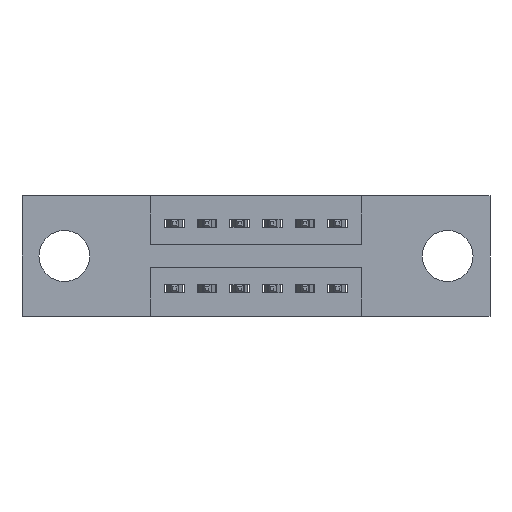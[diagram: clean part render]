
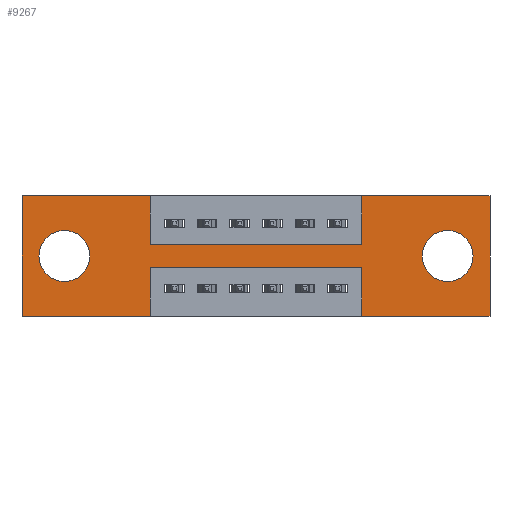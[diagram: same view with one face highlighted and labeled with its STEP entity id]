
A CAD part, front view. The second image highlights one B-rep face of the part: STEP entity #9267.
In plain terms, the highlighted planar face has unit normal (0, -1, 0).
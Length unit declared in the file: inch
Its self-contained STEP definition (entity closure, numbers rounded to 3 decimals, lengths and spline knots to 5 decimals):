
#48 = EDGE_CURVE ( 'NONE', #7557, #5748, #2811, .T. ) ;
#67 = VERTEX_POINT ( 'NONE', #7478 ) ;
#99 = CARTESIAN_POINT ( 'NONE',  ( 0.3925, 0., 0. ) ) ;
#115 = ORIENTED_EDGE ( 'NONE', *, *, #48, .F. ) ;
#135 = VERTEX_POINT ( 'NONE', #356 ) ;
#152 = EDGE_CURVE ( 'NONE', #9398, #7229, #5936, .T. ) ;
#356 = CARTESIAN_POINT ( 'NONE',  ( 0., 0., -0.37 ) ) ;
#578 = VERTEX_POINT ( 'NONE', #6180 ) ;
#628 = ORIENTED_EDGE ( 'NONE', *, *, #1467, .F. ) ;
#659 = DIRECTION ( 'NONE',  ( 0., 0., -1. ) ) ;
#693 = VECTOR ( 'NONE', #9551, 39.37008 ) ;
#712 = ORIENTED_EDGE ( 'NONE', *, *, #730, .T. ) ;
#730 = EDGE_CURVE ( 'NONE', #5898, #7509, #4365, .T. ) ;
#741 = VERTEX_POINT ( 'NONE', #99 ) ;
#786 = EDGE_CURVE ( 'NONE', #741, #578, #2182, .T. ) ;
#837 = DIRECTION ( 'NONE',  ( 0., 0., -1. ) ) ;
#884 = VERTEX_POINT ( 'NONE', #7460 ) ;
#1011 = LINE ( 'NONE', #1949, #693 ) ;
#1019 = LINE ( 'NONE', #2818, #8676 ) ;
#1350 = LINE ( 'NONE', #1994, #3423 ) ;
#1365 = VERTEX_POINT ( 'NONE', #2660 ) ;
#1382 = DIRECTION ( 'NONE',  ( 0., 0., 1. ) ) ;
#1467 = EDGE_CURVE ( 'NONE', #1818, #7557, #5525, .T. ) ;
#1524 = ORIENTED_EDGE ( 'NONE', *, *, #2835, .F. ) ;
#1645 = EDGE_CURVE ( 'NONE', #9322, #135, #4578, .T. ) ;
#1724 = CIRCLE ( 'NONE', #9318, 0.078 ) ;
#1818 = VERTEX_POINT ( 'NONE', #3480 ) ;
#1949 = CARTESIAN_POINT ( 'NONE',  ( 0.3925, 0., -0.22 ) ) ;
#1976 = DIRECTION ( 'NONE',  ( 1., 0., 0. ) ) ;
#1994 = CARTESIAN_POINT ( 'NONE',  ( 0.3925, 0., -0.37 ) ) ;
#2040 = DIRECTION ( 'NONE',  ( 1., 0., 0. ) ) ;
#2086 = DIRECTION ( 'NONE',  ( 0., 0., -1. ) ) ;
#2177 = EDGE_CURVE ( 'NONE', #135, #5758, #5167, .T. ) ;
#2182 = LINE ( 'NONE', #6666, #4133 ) ;
#2308 = CARTESIAN_POINT ( 'NONE',  ( 0., 0., 0. ) ) ;
#2323 = EDGE_CURVE ( 'NONE', #67, #9322, #1350, .T. ) ;
#2373 = AXIS2_PLACEMENT_3D ( 'NONE', #4329, #8053, #5105 ) ;
#2604 = LINE ( 'NONE', #6852, #7099 ) ;
#2633 = CARTESIAN_POINT ( 'NONE',  ( 1.435, 0., 0. ) ) ;
#2660 = CARTESIAN_POINT ( 'NONE',  ( 1.0425, 0., -0.22 ) ) ;
#2692 = CARTESIAN_POINT ( 'NONE',  ( 1.0425, 0., 0. ) ) ;
#2811 = LINE ( 'NONE', #8893, #7665 ) ;
#2818 = CARTESIAN_POINT ( 'NONE',  ( 0., 0., 0. ) ) ;
#2835 = EDGE_CURVE ( 'NONE', #6973, #884, #2604, .T. ) ;
#2857 = ORIENTED_EDGE ( 'NONE', *, *, #4338, .F. ) ;
#2935 = ORIENTED_EDGE ( 'NONE', *, *, #786, .F. ) ;
#2946 = DIRECTION ( 'NONE',  ( 0., 0., 1. ) ) ;
#3013 = EDGE_CURVE ( 'NONE', #7509, #5898, #3643, .T. ) ;
#3135 = LINE ( 'NONE', #7238, #6815 ) ;
#3232 = ORIENTED_EDGE ( 'NONE', *, *, #7795, .F. ) ;
#3386 = CARTESIAN_POINT ( 'NONE',  ( 1.305, 0., -0.107 ) ) ;
#3423 = VECTOR ( 'NONE', #2086, 39.37008 ) ;
#3480 = CARTESIAN_POINT ( 'NONE',  ( 1.0425, 0., -0.15 ) ) ;
#3643 = CIRCLE ( 'NONE', #6067, 0.078 ) ;
#3680 = DIRECTION ( 'NONE',  ( 0., 1., 0. ) ) ;
#3715 = DIRECTION ( 'NONE',  ( 0., 0., -1. ) ) ;
#3824 = DIRECTION ( 'NONE',  ( -1., 0., 0. ) ) ;
#4133 = VECTOR ( 'NONE', #3715, 39.37008 ) ;
#4143 = ORIENTED_EDGE ( 'NONE', *, *, #2323, .F. ) ;
#4182 = AXIS2_PLACEMENT_3D ( 'NONE', #8421, #3680, #2946 ) ;
#4199 = CARTESIAN_POINT ( 'NONE',  ( 1.435, 0., -0.37 ) ) ;
#4212 = FACE_OUTER_BOUND ( 'NONE', #9157, .T. ) ;
#4271 = ORIENTED_EDGE ( 'NONE', *, *, #2177, .F. ) ;
#4310 = CARTESIAN_POINT ( 'NONE',  ( 0.3925, 0., -0.15 ) ) ;
#4329 = CARTESIAN_POINT ( 'NONE',  ( 0., 0., -0.37 ) ) ;
#4333 = FACE_BOUND ( 'NONE', #7493, .T. ) ;
#4338 = EDGE_CURVE ( 'NONE', #884, #1365, #7189, .T. ) ;
#4365 = CIRCLE ( 'NONE', #4182, 0.078 ) ;
#4370 = VECTOR ( 'NONE', #2040, 39.37008 ) ;
#4402 = ORIENTED_EDGE ( 'NONE', *, *, #6558, .F. ) ;
#4446 = DIRECTION ( 'NONE',  ( 1., 0., 0. ) ) ;
#4565 = DIRECTION ( 'NONE',  ( 0., 0., 1. ) ) ;
#4578 = LINE ( 'NONE', #6000, #6687 ) ;
#5061 = FACE_BOUND ( 'NONE', #6332, .T. ) ;
#5105 = DIRECTION ( 'NONE',  ( 0., 0., -1. ) ) ;
#5167 = LINE ( 'NONE', #2308, #6774 ) ;
#5267 = DIRECTION ( 'NONE',  ( 0., 1., 0. ) ) ;
#5436 = CARTESIAN_POINT ( 'NONE',  ( 0.3925, 0., -0.37 ) ) ;
#5525 = LINE ( 'NONE', #6208, #7719 ) ;
#5537 = CARTESIAN_POINT ( 'NONE',  ( 0.13, 0., -0.185 ) ) ;
#5595 = DIRECTION ( 'NONE',  ( 0., 0., 1. ) ) ;
#5748 = VERTEX_POINT ( 'NONE', #2633 ) ;
#5758 = VERTEX_POINT ( 'NONE', #9236 ) ;
#5898 = VERTEX_POINT ( 'NONE', #6348 ) ;
#5936 = CIRCLE ( 'NONE', #8399, 0.078 ) ;
#6000 = CARTESIAN_POINT ( 'NONE',  ( 0., 0., -0.37 ) ) ;
#6039 = EDGE_CURVE ( 'NONE', #5748, #6973, #3135, .T. ) ;
#6067 = AXIS2_PLACEMENT_3D ( 'NONE', #5537, #8468, #5595 ) ;
#6165 = ORIENTED_EDGE ( 'NONE', *, *, #6039, .F. ) ;
#6180 = CARTESIAN_POINT ( 'NONE',  ( 0.3925, 0., -0.15 ) ) ;
#6208 = CARTESIAN_POINT ( 'NONE',  ( 1.0425, 0., 0. ) ) ;
#6332 = EDGE_LOOP ( 'NONE', ( #712, #9542 ) ) ;
#6348 = CARTESIAN_POINT ( 'NONE',  ( 0.13, 0., -0.107 ) ) ;
#6393 = VECTOR ( 'NONE', #1382, 39.37008 ) ;
#6468 = LINE ( 'NONE', #4310, #4370 ) ;
#6513 = ORIENTED_EDGE ( 'NONE', *, *, #1645, .F. ) ;
#6543 = EDGE_CURVE ( 'NONE', #578, #1818, #6468, .T. ) ;
#6558 = EDGE_CURVE ( 'NONE', #5758, #741, #1019, .T. ) ;
#6666 = CARTESIAN_POINT ( 'NONE',  ( 0.3925, 0., 0. ) ) ;
#6687 = VECTOR ( 'NONE', #3824, 39.37008 ) ;
#6712 = EDGE_CURVE ( 'NONE', #7229, #9398, #1724, .T. ) ;
#6774 = VECTOR ( 'NONE', #4565, 39.37008 ) ;
#6815 = VECTOR ( 'NONE', #7306, 39.37008 ) ;
#6852 = CARTESIAN_POINT ( 'NONE',  ( 0., 0., -0.37 ) ) ;
#6874 = DIRECTION ( 'NONE',  ( 0., 0., 1. ) ) ;
#6973 = VERTEX_POINT ( 'NONE', #4199 ) ;
#7099 = VECTOR ( 'NONE', #8408, 39.37008 ) ;
#7189 = LINE ( 'NONE', #8746, #6393 ) ;
#7229 = VERTEX_POINT ( 'NONE', #8800 ) ;
#7238 = CARTESIAN_POINT ( 'NONE',  ( 1.435, 0., 0. ) ) ;
#7306 = DIRECTION ( 'NONE',  ( 0., 0., -1. ) ) ;
#7351 = DIRECTION ( 'NONE',  ( 0., 1., 0. ) ) ;
#7460 = CARTESIAN_POINT ( 'NONE',  ( 1.0425, 0., -0.37 ) ) ;
#7478 = CARTESIAN_POINT ( 'NONE',  ( 0.3925, 0., -0.22 ) ) ;
#7493 = EDGE_LOOP ( 'NONE', ( #9545, #8332 ) ) ;
#7509 = VERTEX_POINT ( 'NONE', #9256 ) ;
#7520 = ORIENTED_EDGE ( 'NONE', *, *, #6543, .F. ) ;
#7557 = VERTEX_POINT ( 'NONE', #2692 ) ;
#7665 = VECTOR ( 'NONE', #4446, 39.37008 ) ;
#7719 = VECTOR ( 'NONE', #6874, 39.37008 ) ;
#7795 = EDGE_CURVE ( 'NONE', #1365, #67, #1011, .T. ) ;
#8053 = DIRECTION ( 'NONE',  ( 0., -1., 0. ) ) ;
#8332 = ORIENTED_EDGE ( 'NONE', *, *, #6712, .T. ) ;
#8399 = AXIS2_PLACEMENT_3D ( 'NONE', #8961, #5267, #837 ) ;
#8408 = DIRECTION ( 'NONE',  ( -1., 0., 0. ) ) ;
#8421 = CARTESIAN_POINT ( 'NONE',  ( 0.13, 0., -0.185 ) ) ;
#8468 = DIRECTION ( 'NONE',  ( 0., 1., 0. ) ) ;
#8676 = VECTOR ( 'NONE', #1976, 39.37008 ) ;
#8746 = CARTESIAN_POINT ( 'NONE',  ( 1.0425, 0., -0.37 ) ) ;
#8799 = CARTESIAN_POINT ( 'NONE',  ( 1.305, 0., -0.185 ) ) ;
#8800 = CARTESIAN_POINT ( 'NONE',  ( 1.305, 0., -0.263 ) ) ;
#8893 = CARTESIAN_POINT ( 'NONE',  ( 0., 0., 0. ) ) ;
#8961 = CARTESIAN_POINT ( 'NONE',  ( 1.305, 0., -0.185 ) ) ;
#9157 = EDGE_LOOP ( 'NONE', ( #4143, #3232, #2857, #1524, #6165, #115, #628, #7520, #2935, #4402, #4271, #6513 ) ) ;
#9236 = CARTESIAN_POINT ( 'NONE',  ( 0., 0., 0. ) ) ;
#9256 = CARTESIAN_POINT ( 'NONE',  ( 0.13, 0., -0.263 ) ) ;
#9267 = ADVANCED_FACE ( 'NONE', ( #4333, #5061, #4212 ), #9529, .T. ) ;
#9318 = AXIS2_PLACEMENT_3D ( 'NONE', #8799, #7351, #659 ) ;
#9322 = VERTEX_POINT ( 'NONE', #5436 ) ;
#9398 = VERTEX_POINT ( 'NONE', #3386 ) ;
#9529 = PLANE ( 'NONE',  #2373 ) ;
#9542 = ORIENTED_EDGE ( 'NONE', *, *, #3013, .T. ) ;
#9545 = ORIENTED_EDGE ( 'NONE', *, *, #152, .T. ) ;
#9551 = DIRECTION ( 'NONE',  ( -1., 0., 0. ) ) ;
